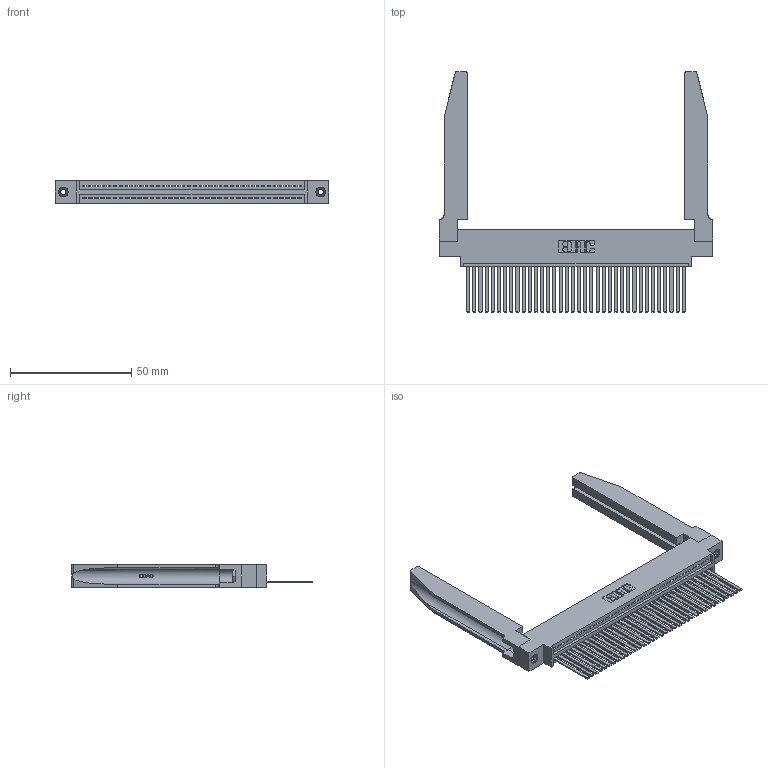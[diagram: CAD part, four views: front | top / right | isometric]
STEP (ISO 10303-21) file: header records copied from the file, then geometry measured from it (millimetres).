
FILE_DESCRIPTION (( 'STEP AP203' ), '1' );
FILE_NAME ('345-036-544-678.STEP', '2019-10-07T23:55:26', ( '' ), ( '' ), 'SwSTEP 2.0', 'SolidWorks 2016', '' );
FILE_SCHEMA (( 'CONFIG_CONTROL_DESIGN' ));
Length unit declared in the file: inch
Products named in the file (5): 345-292-001_345-293-144; 345-250-001_345-250-001-102; 345-220-078_345-220-078; 345-036-544-678; 345 Part_0.170 Offset - 0.156 Dia-TH
Assembly tree (41 placements, depth 2):
  345-036-544-678
    345 Part_0.170 Offset - 0.156 Dia-TH
    345-292-001_345-293-144  x36
    345-250-001_345-250-001-102  x2
    345-220-078_345-220-078  x2
Bounding box: 112.67 x 99.24 x 9.4 mm (x, y, z)
Volume: 18726.8 mm3; surface area: 22702.2 mm2
Topology: 41 solids, 41 shells, 2236 faces, 6649 edges, 4374 vertices
Faces by surface type: plane 1522, cylinder 662, bspline 36, cone 12, torus 4
Entity records: 32590 total; most frequent: CARTESIAN_POINT 6543, ORIENTED_EDGE 5410, DIRECTION 4727, EDGE_CURVE 2705, VECTOR 2339, LINE 2339, VERTEX_POINT 1796, AXIS2_PLACEMENT_3D 1194
